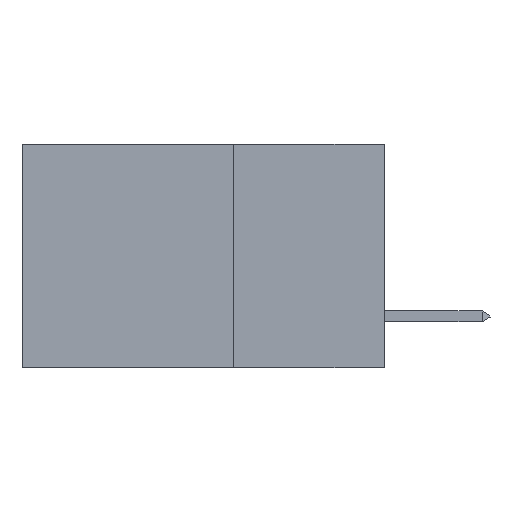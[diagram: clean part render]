
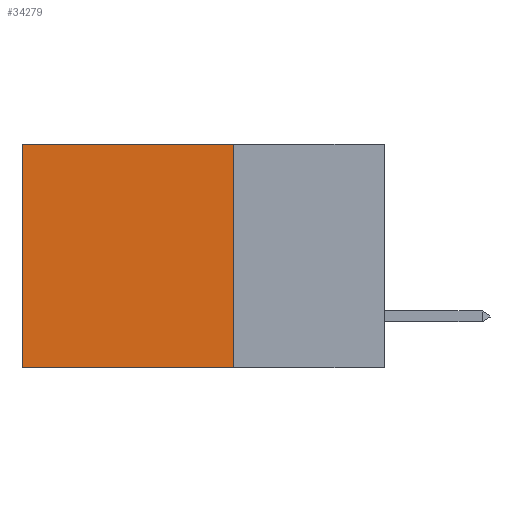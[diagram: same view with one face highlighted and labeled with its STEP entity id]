
A CAD part, left-side view. The second image highlights one B-rep face of the part: STEP entity #34279.
In plain terms, the highlighted planar face has unit normal (-1, 0, 0).
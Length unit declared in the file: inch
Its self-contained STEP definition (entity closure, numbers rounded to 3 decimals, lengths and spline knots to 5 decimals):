
#158 = CARTESIAN_POINT ( 'NONE',  ( 0.2875, 0.25, -0.37 ) ) ;
#269 = LINE ( 'NONE', #39132, #28550 ) ;
#1662 = VERTEX_POINT ( 'NONE', #7647 ) ;
#4425 = FACE_OUTER_BOUND ( 'NONE', #15504, .T. ) ;
#5734 = ORIENTED_EDGE ( 'NONE', *, *, #7766, .T. ) ;
#6672 = LINE ( 'NONE', #29962, #35796 ) ;
#7647 = CARTESIAN_POINT ( 'NONE',  ( 0.2875, 0.6, -0.37 ) ) ;
#7680 = LINE ( 'NONE', #7891, #36791 ) ;
#7766 = EDGE_CURVE ( 'NONE', #43685, #10072, #7680, .T. ) ;
#7778 = VERTEX_POINT ( 'NONE', #158 ) ;
#7891 = CARTESIAN_POINT ( 'NONE',  ( 0.2875, 0.25, 0. ) ) ;
#7896 = DIRECTION ( 'NONE',  ( 1., 0., 0. ) ) ;
#10072 = VERTEX_POINT ( 'NONE', #45466 ) ;
#12355 = PLANE ( 'NONE',  #42267 ) ;
#12507 = CARTESIAN_POINT ( 'NONE',  ( 0.2875, 0.25, 0. ) ) ;
#15504 = EDGE_LOOP ( 'NONE', ( #43368, #41858, #22818, #5734 ) ) ;
#18271 = EDGE_CURVE ( 'NONE', #10072, #1662, #31814, .T. ) ;
#22818 = ORIENTED_EDGE ( 'NONE', *, *, #32839, .F. ) ;
#23643 = DIRECTION ( 'NONE',  ( 0., 0., -1. ) ) ;
#25823 = VECTOR ( 'NONE', #42586, 39.37008 ) ;
#27641 = CARTESIAN_POINT ( 'NONE',  ( 0.2875, 0.6, 0. ) ) ;
#28550 = VECTOR ( 'NONE', #42934, 39.37008 ) ;
#29962 = CARTESIAN_POINT ( 'NONE',  ( 0.2875, 0.25, -0.37 ) ) ;
#31814 = LINE ( 'NONE', #27641, #25823 ) ;
#32012 = EDGE_CURVE ( 'NONE', #7778, #1662, #6672, .T. ) ;
#32839 = EDGE_CURVE ( 'NONE', #43685, #7778, #269, .T. ) ;
#34279 = ADVANCED_FACE ( 'NONE', ( #4425 ), #12355, .F. ) ;
#35796 = VECTOR ( 'NONE', #36787, 39.37008 ) ;
#36787 = DIRECTION ( 'NONE',  ( 0., 1., 0. ) ) ;
#36791 = VECTOR ( 'NONE', #37951, 39.37008 ) ;
#37951 = DIRECTION ( 'NONE',  ( 0., 1., 0. ) ) ;
#39132 = CARTESIAN_POINT ( 'NONE',  ( 0.2875, 0.25, 0. ) ) ;
#41858 = ORIENTED_EDGE ( 'NONE', *, *, #32012, .F. ) ;
#42267 = AXIS2_PLACEMENT_3D ( 'NONE', #42400, #7896, #23643 ) ;
#42400 = CARTESIAN_POINT ( 'NONE',  ( 0.2875, 0.25, 0. ) ) ;
#42586 = DIRECTION ( 'NONE',  ( 0., 0., -1. ) ) ;
#42934 = DIRECTION ( 'NONE',  ( 0., 0., -1. ) ) ;
#43368 = ORIENTED_EDGE ( 'NONE', *, *, #18271, .T. ) ;
#43685 = VERTEX_POINT ( 'NONE', #12507 ) ;
#45466 = CARTESIAN_POINT ( 'NONE',  ( 0.2875, 0.6, 0. ) ) ;
